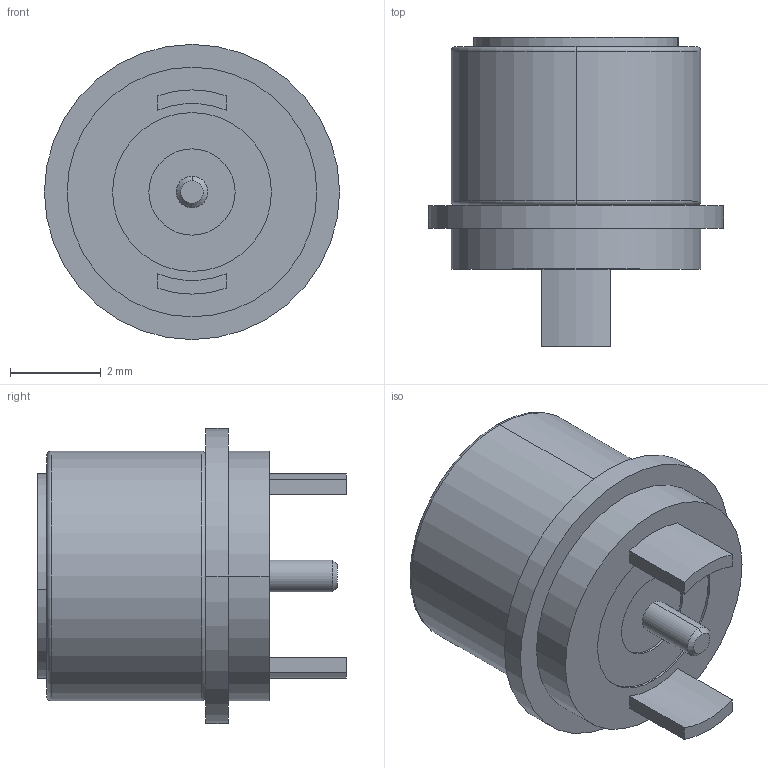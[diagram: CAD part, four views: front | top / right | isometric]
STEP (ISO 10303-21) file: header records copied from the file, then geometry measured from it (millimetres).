
FILE_DESCRIPTION (( 'STEP AP203' ), '1' );
FILE_NAME ('685-A02222021A1.STEP', '2023-02-13T12:35:55', ( 'Magnum' ), ( '' ), 'SwSTEP 2.0', 'SolidWorks 2020', '' );
FILE_SCHEMA (( 'CONFIG_CONTROL_DESIGN' ));
Length unit declared in the file: millimetre
Products named in the file (1): 685-A02222021A1
Bounding box: 6.5 x 6.8 x 6.5 mm (x, y, z)
Volume: 121.7 mm3; surface area: 243.7 mm2
Topology: 2 solids, 3 shells, 66 faces, 138 edges, 87 vertices
Faces by surface type: cylinder 30, plane 20, torus 10, cone 4, sphere 2
Entity records: 1849 total; most frequent: DIRECTION 358, CARTESIAN_POINT 288, ORIENTED_EDGE 270, AXIS2_PLACEMENT_3D 156, EDGE_CURVE 135, CIRCLE 89, VERTEX_POINT 86, EDGE_LOOP 79
